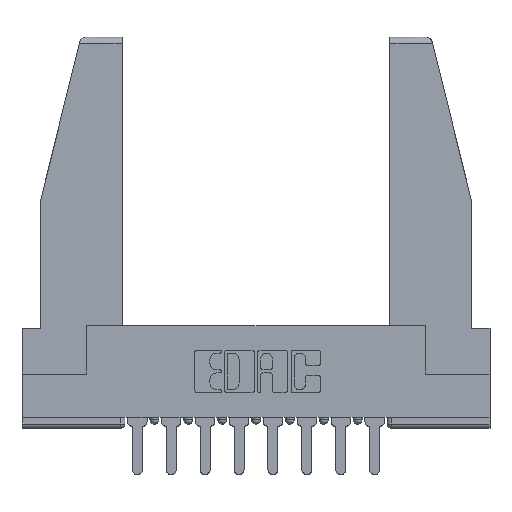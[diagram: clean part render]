
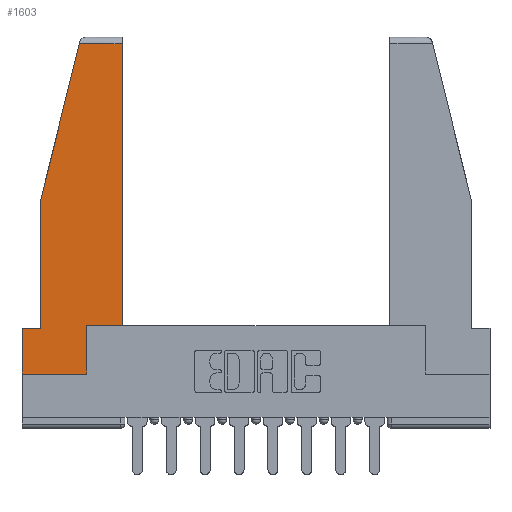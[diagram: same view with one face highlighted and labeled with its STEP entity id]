
A CAD part, top view. The second image highlights one B-rep face of the part: STEP entity #1603.
In plain terms, the highlighted planar face has unit normal (0, 0, 1).
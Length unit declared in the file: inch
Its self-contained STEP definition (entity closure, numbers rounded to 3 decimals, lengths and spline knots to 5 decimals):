
#1159 = CARTESIAN_POINT ( 'NONE',  ( 0.297, 0., 0. ) ) ;
#1175 = DIRECTION ( 'NONE',  ( 1., 0., 0. ) ) ;
#1387 = EDGE_CURVE ( 'NONE', #8138, #7104, #9223, .T. ) ;
#1431 = VECTOR ( 'NONE', #13382, 39.37008 ) ;
#1603 = ADVANCED_FACE ( 'NONE', ( #9403 ), #10227, .T. ) ;
#1617 = CARTESIAN_POINT ( 'NONE',  ( 0.086, 0.8, 0. ) ) ;
#1730 = DIRECTION ( 'NONE',  ( -1., 0., 0. ) ) ;
#1763 = CARTESIAN_POINT ( 'NONE',  ( 0.2636, 1.52, 0. ) ) ;
#1920 = VECTOR ( 'NONE', #7162, 39.37008 ) ;
#1984 = CARTESIAN_POINT ( 'NONE',  ( 0.461, 0.223, 0. ) ) ;
#2123 = EDGE_CURVE ( 'NONE', #12140, #3470, #7871, .T. ) ;
#2271 = ORIENTED_EDGE ( 'NONE', *, *, #5807, .T. ) ;
#2564 = ORIENTED_EDGE ( 'NONE', *, *, #7379, .T. ) ;
#2611 = EDGE_CURVE ( 'NONE', #7104, #5986, #3556, .T. ) ;
#3470 = VERTEX_POINT ( 'NONE', #1763 ) ;
#3556 = LINE ( 'NONE', #1159, #7859 ) ;
#3962 = DIRECTION ( 'NONE',  ( 0., -1., 0. ) ) ;
#3977 = CARTESIAN_POINT ( 'NONE',  ( 0., 0.21, 0. ) ) ;
#4106 = CARTESIAN_POINT ( 'NONE',  ( 0.297, 0.223, 0. ) ) ;
#4395 = CARTESIAN_POINT ( 'NONE',  ( 0.297, 0.223, 0. ) ) ;
#4436 = LINE ( 'NONE', #4395, #13521 ) ;
#4779 = VECTOR ( 'NONE', #9414, 39.37008 ) ;
#4784 = CARTESIAN_POINT ( 'NONE',  ( 0.461, 1.52, 0. ) ) ;
#4789 = LINE ( 'NONE', #9244, #10733 ) ;
#4868 = CARTESIAN_POINT ( 'NONE',  ( 0.461, 0.223, 0. ) ) ;
#4978 = DIRECTION ( 'NONE',  ( 0., 0., 1. ) ) ;
#5198 = ORIENTED_EDGE ( 'NONE', *, *, #2123, .T. ) ;
#5298 = VECTOR ( 'NONE', #6299, 39.37008 ) ;
#5807 = EDGE_CURVE ( 'NONE', #13580, #8138, #4789, .T. ) ;
#5882 = CARTESIAN_POINT ( 'NONE',  ( 0., 1.52, 0. ) ) ;
#5986 = VERTEX_POINT ( 'NONE', #4106 ) ;
#6063 = CARTESIAN_POINT ( 'NONE',  ( 0.086, 0.21, 0. ) ) ;
#6299 = DIRECTION ( 'NONE',  ( 0., -1., 0. ) ) ;
#6320 = EDGE_CURVE ( 'NONE', #12278, #13580, #13523, .T. ) ;
#7104 = VERTEX_POINT ( 'NONE', #9743 ) ;
#7162 = DIRECTION ( 'NONE',  ( -1., 0., 0. ) ) ;
#7379 = EDGE_CURVE ( 'NONE', #3470, #8511, #8075, .T. ) ;
#7553 = VECTOR ( 'NONE', #1730, 39.37008 ) ;
#7623 = EDGE_CURVE ( 'NONE', #5986, #10357, #4436, .T. ) ;
#7850 = CARTESIAN_POINT ( 'NONE',  ( 0.271, 1.55, 0. ) ) ;
#7859 = VECTOR ( 'NONE', #8577, 39.37008 ) ;
#7871 = LINE ( 'NONE', #5882, #7553 ) ;
#8075 = LINE ( 'NONE', #7850, #8405 ) ;
#8138 = VERTEX_POINT ( 'NONE', #13652 ) ;
#8388 = ORIENTED_EDGE ( 'NONE', *, *, #11225, .T. ) ;
#8405 = VECTOR ( 'NONE', #10033, 39.37008 ) ;
#8447 = CARTESIAN_POINT ( 'NONE',  ( 0.086, 0.8, 0. ) ) ;
#8511 = VERTEX_POINT ( 'NONE', #1617 ) ;
#8577 = DIRECTION ( 'NONE',  ( 0., 1., 0. ) ) ;
#8813 = ORIENTED_EDGE ( 'NONE', *, *, #11741, .T. ) ;
#8956 = CARTESIAN_POINT ( 'NONE',  ( 0., 0., 0. ) ) ;
#9137 = ORIENTED_EDGE ( 'NONE', *, *, #1387, .T. ) ;
#9223 = LINE ( 'NONE', #8956, #1431 ) ;
#9244 = CARTESIAN_POINT ( 'NONE',  ( 0., 0.21, 0. ) ) ;
#9403 = FACE_OUTER_BOUND ( 'NONE', #9741, .T. ) ;
#9406 = LINE ( 'NONE', #1984, #4779 ) ;
#9414 = DIRECTION ( 'NONE',  ( 0., 1., 0. ) ) ;
#9741 = EDGE_LOOP ( 'NONE', ( #8813, #5198, #2564, #8388, #11689, #2271, #9137, #12309, #12581 ) ) ;
#9743 = CARTESIAN_POINT ( 'NONE',  ( 0.297, 0., 0. ) ) ;
#10033 = DIRECTION ( 'NONE',  ( -0.239, -0.971, 0. ) ) ;
#10174 = CARTESIAN_POINT ( 'NONE',  ( 0., 0.21, 0. ) ) ;
#10227 = PLANE ( 'NONE',  #12628 ) ;
#10357 = VERTEX_POINT ( 'NONE', #4868 ) ;
#10733 = VECTOR ( 'NONE', #3962, 39.37008 ) ;
#11225 = EDGE_CURVE ( 'NONE', #8511, #12278, #13392, .T. ) ;
#11689 = ORIENTED_EDGE ( 'NONE', *, *, #6320, .T. ) ;
#11741 = EDGE_CURVE ( 'NONE', #10357, #12140, #9406, .T. ) ;
#12140 = VERTEX_POINT ( 'NONE', #4784 ) ;
#12278 = VERTEX_POINT ( 'NONE', #6063 ) ;
#12309 = ORIENTED_EDGE ( 'NONE', *, *, #2611, .T. ) ;
#12353 = DIRECTION ( 'NONE',  ( 1., 0., 0. ) ) ;
#12581 = ORIENTED_EDGE ( 'NONE', *, *, #7623, .T. ) ;
#12628 = AXIS2_PLACEMENT_3D ( 'NONE', #13553, #4978, #12353 ) ;
#13382 = DIRECTION ( 'NONE',  ( 1., 0., 0. ) ) ;
#13392 = LINE ( 'NONE', #8447, #5298 ) ;
#13521 = VECTOR ( 'NONE', #1175, 39.37008 ) ;
#13523 = LINE ( 'NONE', #3977, #1920 ) ;
#13553 = CARTESIAN_POINT ( 'NONE',  ( 0., 0., 0. ) ) ;
#13580 = VERTEX_POINT ( 'NONE', #10174 ) ;
#13652 = CARTESIAN_POINT ( 'NONE',  ( 0., 0., 0. ) ) ;
